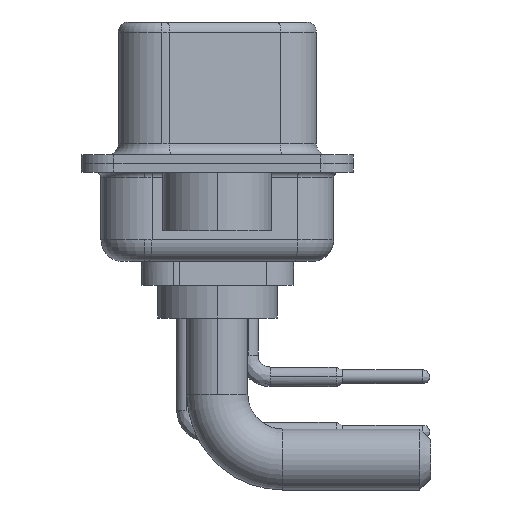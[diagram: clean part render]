
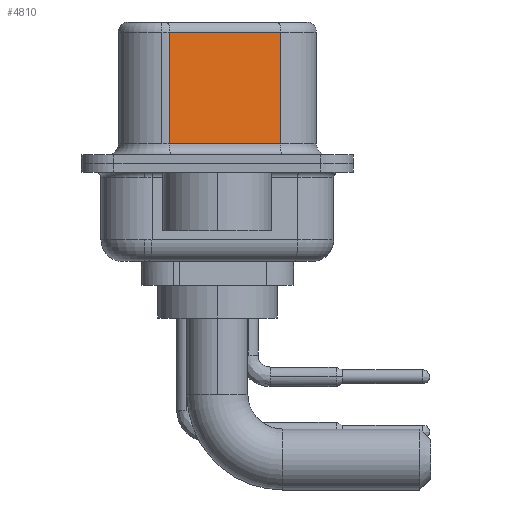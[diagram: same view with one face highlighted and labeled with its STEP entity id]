
A CAD part, left-side view. The second image highlights one B-rep face of the part: STEP entity #4810.
In plain terms, the highlighted planar face has unit normal (-0.985, -0.174, 0).
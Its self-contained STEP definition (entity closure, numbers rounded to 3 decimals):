
#171 = LINE ( 'NONE', #21930, #18003 ) ;
#299 = CARTESIAN_POINT ( 'NONE',  ( 3.68, 2.203, 6.02 ) ) ;
#375 = ORIENTED_EDGE ( 'NONE', *, *, #11241, .T. ) ;
#861 = AXIS2_PLACEMENT_3D ( 'NONE', #8204, #15143, #3091 ) ;
#901 = DIRECTION ( 'NONE',  ( -0.174, 0.985, 0. ) ) ;
#1368 = VECTOR ( 'NONE', #901, 1000. ) ;
#2303 = CARTESIAN_POINT ( 'NONE',  ( 3.68, 2.203, 0.9 ) ) ;
#3091 = DIRECTION ( 'NONE',  ( -0.174, 0.985, 0. ) ) ;
#3143 = VERTEX_POINT ( 'NONE', #299 ) ;
#3928 = CARTESIAN_POINT ( 'NONE',  ( 3.68, 2.203, 6.52 ) ) ;
#4810 = ADVANCED_FACE ( 'NONE', ( #16841 ), #21962, .F. ) ;
#5298 = DIRECTION ( 'NONE',  ( 0.174, -0.985, 0. ) ) ;
#7594 = ORIENTED_EDGE ( 'NONE', *, *, #14489, .F. ) ;
#8160 = DIRECTION ( 'NONE',  ( 0., 0., -1. ) ) ;
#8204 = CARTESIAN_POINT ( 'NONE',  ( 4.58, -2.897, 6.52 ) ) ;
#8596 = VERTEX_POINT ( 'NONE', #2303 ) ;
#9394 = VECTOR ( 'NONE', #21214, 1000. ) ;
#9549 = LINE ( 'NONE', #21929, #1368 ) ;
#10529 = EDGE_CURVE ( 'NONE', #12562, #3143, #9549, .T. ) ;
#11241 = EDGE_CURVE ( 'NONE', #8596, #20488, #171, .T. ) ;
#11316 = VECTOR ( 'NONE', #8160, 1000. ) ;
#11815 = LINE ( 'NONE', #15428, #11316 ) ;
#12562 = VERTEX_POINT ( 'NONE', #22282 ) ;
#14026 = ORIENTED_EDGE ( 'NONE', *, *, #18521, .T. ) ;
#14489 = EDGE_CURVE ( 'NONE', #12562, #20488, #11815, .T. ) ;
#15143 = DIRECTION ( 'NONE',  ( 0.985, 0.174, 0. ) ) ;
#15428 = CARTESIAN_POINT ( 'NONE',  ( 4.58, -2.897, 6.52 ) ) ;
#15977 = LINE ( 'NONE', #3928, #9394 ) ;
#16459 = EDGE_LOOP ( 'NONE', ( #7594, #17266, #14026, #375 ) ) ;
#16841 = FACE_OUTER_BOUND ( 'NONE', #16459, .T. ) ;
#17266 = ORIENTED_EDGE ( 'NONE', *, *, #10529, .T. ) ;
#18003 = VECTOR ( 'NONE', #5298, 1000. ) ;
#18521 = EDGE_CURVE ( 'NONE', #3143, #8596, #15977, .T. ) ;
#20488 = VERTEX_POINT ( 'NONE', #21087 ) ;
#21087 = CARTESIAN_POINT ( 'NONE',  ( 4.58, -2.897, 0.9 ) ) ;
#21214 = DIRECTION ( 'NONE',  ( 0., 0., -1. ) ) ;
#21929 = CARTESIAN_POINT ( 'NONE',  ( 4.58, -2.897, 6.02 ) ) ;
#21930 = CARTESIAN_POINT ( 'NONE',  ( 4.58, -2.897, 0.9 ) ) ;
#21962 = PLANE ( 'NONE',  #861 ) ;
#22282 = CARTESIAN_POINT ( 'NONE',  ( 4.58, -2.897, 6.02 ) ) ;
